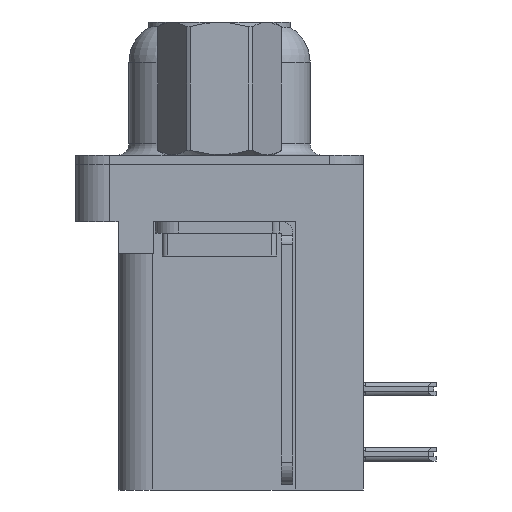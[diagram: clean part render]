
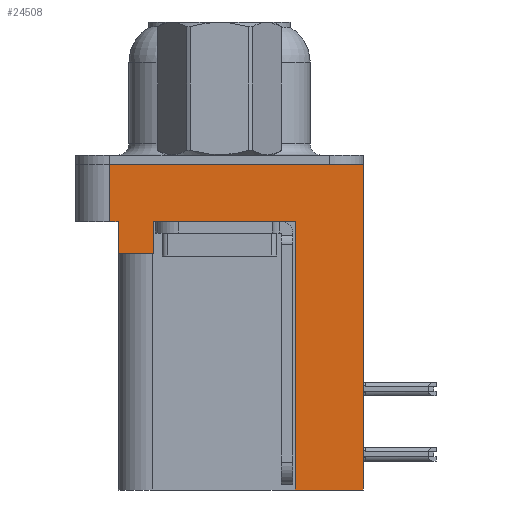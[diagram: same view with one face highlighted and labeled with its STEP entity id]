
A CAD part, left-side view. The second image highlights one B-rep face of the part: STEP entity #24508.
In plain terms, the highlighted planar face has unit normal (-1, 0, 0).
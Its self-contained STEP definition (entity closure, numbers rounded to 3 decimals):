
#681 = CARTESIAN_POINT ( 'NONE',  ( -2.91, -6.275, -2.5 ) ) ;
#988 = CARTESIAN_POINT ( 'NONE',  ( -2.91, -6.275, -2.5 ) ) ;
#1678 = EDGE_CURVE ( 'NONE', #36733, #27535, #21898, .T. ) ;
#2271 = CARTESIAN_POINT ( 'NONE',  ( -2.91, 4.775, 0. ) ) ;
#2561 = ORIENTED_EDGE ( 'NONE', *, *, #19165, .F. ) ;
#3517 = CARTESIAN_POINT ( 'NONE',  ( -2.91, 2.895, -3.9 ) ) ;
#3704 = DIRECTION ( 'NONE',  ( 0., 0., 1. ) ) ;
#4871 = CARTESIAN_POINT ( 'NONE',  ( -2.91, -6.275, -2.5 ) ) ;
#4924 = DIRECTION ( 'NONE',  ( 0., 1., 0. ) ) ;
#5404 = EDGE_CURVE ( 'NONE', #27224, #6771, #39241, .T. ) ;
#5715 = LINE ( 'NONE', #18821, #34734 ) ;
#5893 = VECTOR ( 'NONE', #16954, 1000. ) ;
#6332 = DIRECTION ( 'NONE',  ( 0., -1., 0. ) ) ;
#6602 = CARTESIAN_POINT ( 'NONE',  ( -2.91, 4.425, -3.9 ) ) ;
#6771 = VERTEX_POINT ( 'NONE', #26806 ) ;
#7026 = LINE ( 'NONE', #6602, #39564 ) ;
#7415 = LINE ( 'NONE', #29478, #15941 ) ;
#8096 = ORIENTED_EDGE ( 'NONE', *, *, #38598, .T. ) ;
#8387 = EDGE_CURVE ( 'NONE', #10562, #15002, #5715, .T. ) ;
#8942 = CARTESIAN_POINT ( 'NONE',  ( -2.91, -6.275, 0. ) ) ;
#10562 = VERTEX_POINT ( 'NONE', #2271 ) ;
#10728 = ORIENTED_EDGE ( 'NONE', *, *, #25918, .F. ) ;
#10907 = VECTOR ( 'NONE', #12955, 1000. ) ;
#11740 = LINE ( 'NONE', #24423, #28060 ) ;
#11997 = CARTESIAN_POINT ( 'NONE',  ( -2.91, -3.295, -2.5 ) ) ;
#12196 = VERTEX_POINT ( 'NONE', #11997 ) ;
#12345 = LINE ( 'NONE', #15642, #14670 ) ;
#12955 = DIRECTION ( 'NONE',  ( 0., 0., 1. ) ) ;
#13139 = EDGE_CURVE ( 'NONE', #17075, #15002, #13157, .T. ) ;
#13157 = LINE ( 'NONE', #681, #10907 ) ;
#13683 = DIRECTION ( 'NONE',  ( 0., -1., 0. ) ) ;
#14670 = VECTOR ( 'NONE', #41064, 1000. ) ;
#15002 = VERTEX_POINT ( 'NONE', #8942 ) ;
#15063 = VECTOR ( 'NONE', #22224, 1000. ) ;
#15117 = CARTESIAN_POINT ( 'NONE',  ( -2.91, 4.425, -2.5 ) ) ;
#15365 = LINE ( 'NONE', #21618, #15063 ) ;
#15600 = VERTEX_POINT ( 'NONE', #35705 ) ;
#15642 = CARTESIAN_POINT ( 'NONE',  ( -2.91, -3.295, -14.2 ) ) ;
#15941 = VECTOR ( 'NONE', #4924, 1000. ) ;
#16750 = CARTESIAN_POINT ( 'NONE',  ( -2.91, 2.895, -3.9 ) ) ;
#16954 = DIRECTION ( 'NONE',  ( 0., 0., 1. ) ) ;
#17075 = VERTEX_POINT ( 'NONE', #20274 ) ;
#17509 = EDGE_CURVE ( 'NONE', #15600, #27535, #7026, .T. ) ;
#17860 = ORIENTED_EDGE ( 'NONE', *, *, #13139, .T. ) ;
#17953 = FACE_OUTER_BOUND ( 'NONE', #24756, .T. ) ;
#18178 = DIRECTION ( 'NONE',  ( 0., 0., 1. ) ) ;
#18821 = CARTESIAN_POINT ( 'NONE',  ( -2.91, -6.275, 0. ) ) ;
#19165 = EDGE_CURVE ( 'NONE', #17075, #21713, #15365, .T. ) ;
#19407 = CARTESIAN_POINT ( 'NONE',  ( -2.91, 4.775, -2.5 ) ) ;
#19514 = ORIENTED_EDGE ( 'NONE', *, *, #36593, .F. ) ;
#20098 = CARTESIAN_POINT ( 'NONE',  ( -2.91, -3.295, -14.2 ) ) ;
#20274 = CARTESIAN_POINT ( 'NONE',  ( -2.91, -6.275, -14.2 ) ) ;
#20696 = VECTOR ( 'NONE', #32053, 1000. ) ;
#21618 = CARTESIAN_POINT ( 'NONE',  ( -2.91, -3.295, -14.2 ) ) ;
#21713 = VERTEX_POINT ( 'NONE', #20098 ) ;
#21839 = ORIENTED_EDGE ( 'NONE', *, *, #8387, .F. ) ;
#21898 = LINE ( 'NONE', #32882, #20696 ) ;
#22224 = DIRECTION ( 'NONE',  ( 0., 1., 0. ) ) ;
#22849 = LINE ( 'NONE', #988, #30820 ) ;
#23530 = ORIENTED_EDGE ( 'NONE', *, *, #35411, .F. ) ;
#23623 = ORIENTED_EDGE ( 'NONE', *, *, #5404, .T. ) ;
#24000 = DIRECTION ( 'NONE',  ( -1., 0., 0. ) ) ;
#24423 = CARTESIAN_POINT ( 'NONE',  ( -2.91, 4.775, -2.5 ) ) ;
#24508 = ADVANCED_FACE ( 'NONE', ( #17953 ), #26917, .T. ) ;
#24756 = EDGE_LOOP ( 'NONE', ( #21839, #19514, #35707, #35835, #10728, #23623, #8096, #23530, #2561, #17860 ) ) ;
#25918 = EDGE_CURVE ( 'NONE', #27224, #15600, #7415, .T. ) ;
#26806 = CARTESIAN_POINT ( 'NONE',  ( -2.91, 2.895, -2.5 ) ) ;
#26917 = PLANE ( 'NONE',  #28506 ) ;
#27224 = VERTEX_POINT ( 'NONE', #3517 ) ;
#27535 = VERTEX_POINT ( 'NONE', #15117 ) ;
#28060 = VECTOR ( 'NONE', #18178, 1000. ) ;
#28506 = AXIS2_PLACEMENT_3D ( 'NONE', #4871, #24000, #36085 ) ;
#29478 = CARTESIAN_POINT ( 'NONE',  ( -2.91, 4.425, -3.9 ) ) ;
#30820 = VECTOR ( 'NONE', #13683, 1000. ) ;
#32053 = DIRECTION ( 'NONE',  ( 0., -1., 0. ) ) ;
#32882 = CARTESIAN_POINT ( 'NONE',  ( -2.91, -6.275, -2.5 ) ) ;
#34734 = VECTOR ( 'NONE', #6332, 1000. ) ;
#35411 = EDGE_CURVE ( 'NONE', #21713, #12196, #12345, .T. ) ;
#35705 = CARTESIAN_POINT ( 'NONE',  ( -2.91, 4.425, -3.9 ) ) ;
#35707 = ORIENTED_EDGE ( 'NONE', *, *, #1678, .T. ) ;
#35835 = ORIENTED_EDGE ( 'NONE', *, *, #17509, .F. ) ;
#36085 = DIRECTION ( 'NONE',  ( 0., 0., 1. ) ) ;
#36593 = EDGE_CURVE ( 'NONE', #36733, #10562, #11740, .T. ) ;
#36733 = VERTEX_POINT ( 'NONE', #19407 ) ;
#38598 = EDGE_CURVE ( 'NONE', #6771, #12196, #22849, .T. ) ;
#39241 = LINE ( 'NONE', #16750, #5893 ) ;
#39564 = VECTOR ( 'NONE', #3704, 1000. ) ;
#41064 = DIRECTION ( 'NONE',  ( 0., 0., 1. ) ) ;
